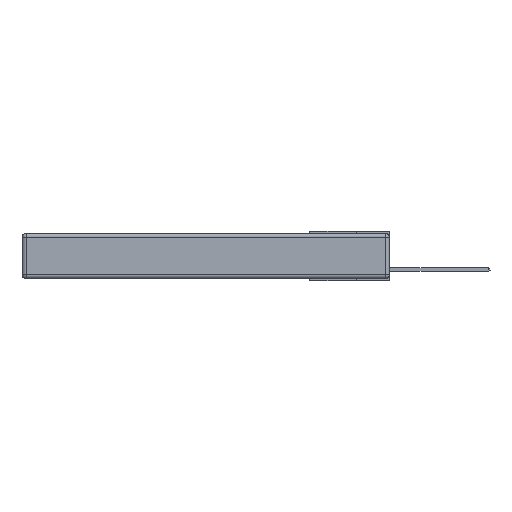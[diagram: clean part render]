
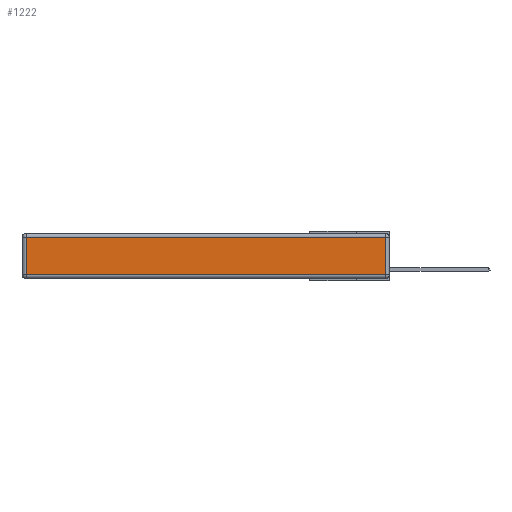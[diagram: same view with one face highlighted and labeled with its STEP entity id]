
A CAD part, left-side view. The second image highlights one B-rep face of the part: STEP entity #1222.
In plain terms, the highlighted planar face has unit normal (-1, 0, 0).
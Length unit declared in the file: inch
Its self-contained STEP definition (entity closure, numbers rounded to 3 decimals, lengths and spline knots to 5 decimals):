
#328 = EDGE_LOOP ( 'NONE', ( #22418, #13477, #18121, #4242 ) ) ;
#439 = EDGE_CURVE ( 'NONE', #7752, #2122, #3517, .T. ) ;
#1103 = LINE ( 'NONE', #21112, #8288 ) ;
#1222 = ADVANCED_FACE ( 'NONE', ( #19570 ), #15333, .T. ) ;
#2122 = VERTEX_POINT ( 'NONE', #32747 ) ;
#3517 = LINE ( 'NONE', #4319, #16822 ) ;
#4242 = ORIENTED_EDGE ( 'NONE', *, *, #9438, .T. ) ;
#4278 = VECTOR ( 'NONE', #25686, 39.37008 ) ;
#4319 = CARTESIAN_POINT ( 'NONE',  ( 0., 0.03, -0.343 ) ) ;
#4714 = LINE ( 'NONE', #12374, #7099 ) ;
#5155 = CARTESIAN_POINT ( 'NONE',  ( 0., 2.72, -0.03 ) ) ;
#5682 = DIRECTION ( 'NONE',  ( 0., 1., 0. ) ) ;
#7099 = VECTOR ( 'NONE', #25232, 39.37008 ) ;
#7752 = VERTEX_POINT ( 'NONE', #8045 ) ;
#8045 = CARTESIAN_POINT ( 'NONE',  ( 0., 0.03, -0.313 ) ) ;
#8288 = VECTOR ( 'NONE', #5682, 39.37008 ) ;
#9334 = DIRECTION ( 'NONE',  ( 0., 0., 1. ) ) ;
#9438 = EDGE_CURVE ( 'NONE', #16668, #14925, #4714, .T. ) ;
#10057 = CARTESIAN_POINT ( 'NONE',  ( 0., 0., -0.343 ) ) ;
#10274 = DIRECTION ( 'NONE',  ( 0., 0., 1. ) ) ;
#11084 = LINE ( 'NONE', #22786, #4278 ) ;
#12374 = CARTESIAN_POINT ( 'NONE',  ( 0., 2.72, -0.343 ) ) ;
#13215 = EDGE_CURVE ( 'NONE', #14925, #7752, #11084, .T. ) ;
#13477 = ORIENTED_EDGE ( 'NONE', *, *, #439, .T. ) ;
#14925 = VERTEX_POINT ( 'NONE', #24557 ) ;
#15333 = PLANE ( 'NONE',  #22995 ) ;
#16668 = VERTEX_POINT ( 'NONE', #5155 ) ;
#16822 = VECTOR ( 'NONE', #9334, 39.37008 ) ;
#17998 = EDGE_CURVE ( 'NONE', #2122, #16668, #1103, .T. ) ;
#18121 = ORIENTED_EDGE ( 'NONE', *, *, #17998, .T. ) ;
#19570 = FACE_OUTER_BOUND ( 'NONE', #328, .T. ) ;
#21112 = CARTESIAN_POINT ( 'NONE',  ( 0., 2.75, -0.03 ) ) ;
#22418 = ORIENTED_EDGE ( 'NONE', *, *, #13215, .T. ) ;
#22786 = CARTESIAN_POINT ( 'NONE',  ( 0., 0., -0.313 ) ) ;
#22995 = AXIS2_PLACEMENT_3D ( 'NONE', #10057, #33301, #10274 ) ;
#24557 = CARTESIAN_POINT ( 'NONE',  ( 0., 2.72, -0.313 ) ) ;
#25232 = DIRECTION ( 'NONE',  ( 0., 0., -1. ) ) ;
#25686 = DIRECTION ( 'NONE',  ( 0., -1., 0. ) ) ;
#32747 = CARTESIAN_POINT ( 'NONE',  ( 0., 0.03, -0.03 ) ) ;
#33301 = DIRECTION ( 'NONE',  ( -1., 0., 0. ) ) ;
